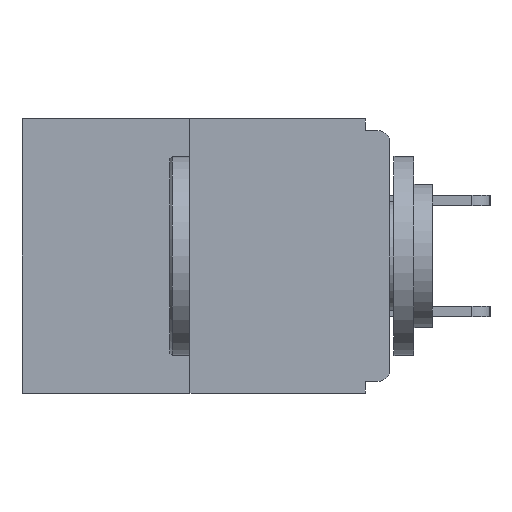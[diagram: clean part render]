
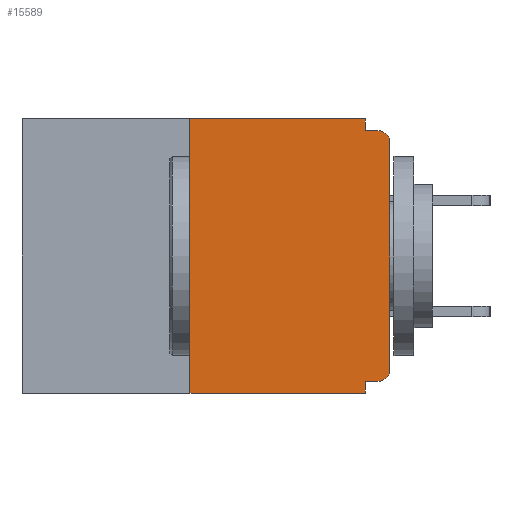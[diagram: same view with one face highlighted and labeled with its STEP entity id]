
A CAD part, left-side view. The second image highlights one B-rep face of the part: STEP entity #15589.
In plain terms, the highlighted planar face has unit normal (-1, 0, 0).
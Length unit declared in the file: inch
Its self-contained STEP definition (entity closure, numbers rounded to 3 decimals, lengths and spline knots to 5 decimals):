
#80 = CARTESIAN_POINT ( 'NONE',  ( 0., 0.031, -0.015 ) ) ;
#157 = VECTOR ( 'NONE', #888, 39.37008 ) ;
#400 = CARTESIAN_POINT ( 'NONE',  ( 0., 0.25, -0.343 ) ) ;
#420 = VERTEX_POINT ( 'NONE', #7724 ) ;
#677 = LINE ( 'NONE', #5619, #21829 ) ;
#743 = ORIENTED_EDGE ( 'NONE', *, *, #17742, .F. ) ;
#871 = AXIS2_PLACEMENT_3D ( 'NONE', #3648, #18218, #20045 ) ;
#888 = DIRECTION ( 'NONE',  ( 0., 1., 0. ) ) ;
#1021 = EDGE_CURVE ( 'NONE', #12493, #19954, #9969, .T. ) ;
#1078 = VERTEX_POINT ( 'NONE', #400 ) ;
#1182 = LINE ( 'NONE', #8046, #20086 ) ;
#1927 = EDGE_CURVE ( 'NONE', #1078, #22953, #1182, .T. ) ;
#2009 = LINE ( 'NONE', #21071, #23211 ) ;
#2284 = DIRECTION ( 'NONE',  ( 0., 0., 1. ) ) ;
#2477 = AXIS2_PLACEMENT_3D ( 'NONE', #3922, #16355, #16504 ) ;
#2522 = AXIS2_PLACEMENT_3D ( 'NONE', #11956, #6520, #19119 ) ;
#2690 = VECTOR ( 'NONE', #9594, 39.37008 ) ;
#3338 = LINE ( 'NONE', #4426, #21393 ) ;
#3648 = CARTESIAN_POINT ( 'NONE',  ( 0., 0.015, -0.03 ) ) ;
#3759 = PLANE ( 'NONE',  #2477 ) ;
#3922 = CARTESIAN_POINT ( 'NONE',  ( 0., 0.46, 0. ) ) ;
#4188 = VERTEX_POINT ( 'NONE', #22396 ) ;
#4380 = CARTESIAN_POINT ( 'NONE',  ( 0., 0., 0. ) ) ;
#4407 = LINE ( 'NONE', #6407, #157 ) ;
#4426 = CARTESIAN_POINT ( 'NONE',  ( 0., 0.46, 0. ) ) ;
#4611 = ORIENTED_EDGE ( 'NONE', *, *, #5428, .T. ) ;
#5428 = EDGE_CURVE ( 'NONE', #420, #12493, #16795, .T. ) ;
#5619 = CARTESIAN_POINT ( 'NONE',  ( 0., 0.25, 0. ) ) ;
#5857 = CARTESIAN_POINT ( 'NONE',  ( 0., 0., -0.015 ) ) ;
#6407 = CARTESIAN_POINT ( 'NONE',  ( 0., 0., -0.328 ) ) ;
#6520 = DIRECTION ( 'NONE',  ( -1., 0., 0. ) ) ;
#6890 = ORIENTED_EDGE ( 'NONE', *, *, #16379, .F. ) ;
#7247 = VERTEX_POINT ( 'NONE', #80 ) ;
#7355 = VECTOR ( 'NONE', #14670, 39.37008 ) ;
#7632 = EDGE_CURVE ( 'NONE', #8099, #22953, #16119, .T. ) ;
#7711 = CARTESIAN_POINT ( 'NONE',  ( 0., 0.031, -0.328 ) ) ;
#7717 = CARTESIAN_POINT ( 'NONE',  ( 0., 0.031, -0.343 ) ) ;
#7724 = CARTESIAN_POINT ( 'NONE',  ( 0., 0., -0.313 ) ) ;
#7818 = EDGE_LOOP ( 'NONE', ( #6890, #14769, #8709, #11489, #743, #15421, #4611, #19420, #20876, #22952 ) ) ;
#8046 = CARTESIAN_POINT ( 'NONE',  ( 0., 0.46, -0.343 ) ) ;
#8099 = VERTEX_POINT ( 'NONE', #7711 ) ;
#8523 = CARTESIAN_POINT ( 'NONE',  ( 0., 0.031, -0.343 ) ) ;
#8709 = ORIENTED_EDGE ( 'NONE', *, *, #1927, .T. ) ;
#9594 = DIRECTION ( 'NONE',  ( 0., 0., 1. ) ) ;
#9792 = DIRECTION ( 'NONE',  ( 0., -1., 0. ) ) ;
#9969 = CIRCLE ( 'NONE', #871, 0.015 ) ;
#10234 = DIRECTION ( 'NONE',  ( 0., 0., -1. ) ) ;
#10933 = FACE_OUTER_BOUND ( 'NONE', #7818, .T. ) ;
#11489 = ORIENTED_EDGE ( 'NONE', *, *, #7632, .F. ) ;
#11716 = CARTESIAN_POINT ( 'NONE',  ( 0., 0.031, 0. ) ) ;
#11956 = CARTESIAN_POINT ( 'NONE',  ( 0., 0.015, -0.313 ) ) ;
#12306 = EDGE_CURVE ( 'NONE', #1078, #14085, #677, .T. ) ;
#12493 = VERTEX_POINT ( 'NONE', #13215 ) ;
#13215 = CARTESIAN_POINT ( 'NONE',  ( 0., 0., -0.03 ) ) ;
#14085 = VERTEX_POINT ( 'NONE', #19715 ) ;
#14670 = DIRECTION ( 'NONE',  ( 0., -1., 0. ) ) ;
#14769 = ORIENTED_EDGE ( 'NONE', *, *, #12306, .F. ) ;
#15261 = DIRECTION ( 'NONE',  ( 0., -1., 0. ) ) ;
#15421 = ORIENTED_EDGE ( 'NONE', *, *, #17247, .T. ) ;
#15589 = ADVANCED_FACE ( 'NONE', ( #10933 ), #3759, .F. ) ;
#16119 = LINE ( 'NONE', #8523, #21759 ) ;
#16355 = DIRECTION ( 'NONE',  ( 1., 0., 0. ) ) ;
#16379 = EDGE_CURVE ( 'NONE', #14085, #23009, #3338, .T. ) ;
#16504 = DIRECTION ( 'NONE',  ( 0., 0., -1. ) ) ;
#16795 = LINE ( 'NONE', #4380, #2690 ) ;
#17247 = EDGE_CURVE ( 'NONE', #4188, #420, #22740, .T. ) ;
#17433 = DIRECTION ( 'NONE',  ( 0., 0., -1. ) ) ;
#17742 = EDGE_CURVE ( 'NONE', #4188, #8099, #4407, .T. ) ;
#18218 = DIRECTION ( 'NONE',  ( -1., 0., 0. ) ) ;
#19119 = DIRECTION ( 'NONE',  ( 0., 0., -1. ) ) ;
#19420 = ORIENTED_EDGE ( 'NONE', *, *, #1021, .T. ) ;
#19437 = EDGE_CURVE ( 'NONE', #23009, #7247, #2009, .T. ) ;
#19715 = CARTESIAN_POINT ( 'NONE',  ( 0., 0.25, 0. ) ) ;
#19954 = VERTEX_POINT ( 'NONE', #21989 ) ;
#20045 = DIRECTION ( 'NONE',  ( 0., 0., -1. ) ) ;
#20086 = VECTOR ( 'NONE', #15261, 39.37008 ) ;
#20876 = ORIENTED_EDGE ( 'NONE', *, *, #21130, .F. ) ;
#21071 = CARTESIAN_POINT ( 'NONE',  ( 0., 0.031, 0. ) ) ;
#21130 = EDGE_CURVE ( 'NONE', #7247, #19954, #22000, .T. ) ;
#21393 = VECTOR ( 'NONE', #9792, 39.37008 ) ;
#21759 = VECTOR ( 'NONE', #10234, 39.37008 ) ;
#21829 = VECTOR ( 'NONE', #2284, 39.37008 ) ;
#21989 = CARTESIAN_POINT ( 'NONE',  ( 0., 0.015, -0.015 ) ) ;
#22000 = LINE ( 'NONE', #5857, #7355 ) ;
#22396 = CARTESIAN_POINT ( 'NONE',  ( 0., 0.015, -0.328 ) ) ;
#22740 = CIRCLE ( 'NONE', #2522, 0.015 ) ;
#22952 = ORIENTED_EDGE ( 'NONE', *, *, #19437, .F. ) ;
#22953 = VERTEX_POINT ( 'NONE', #7717 ) ;
#23009 = VERTEX_POINT ( 'NONE', #11716 ) ;
#23211 = VECTOR ( 'NONE', #17433, 39.37008 ) ;
